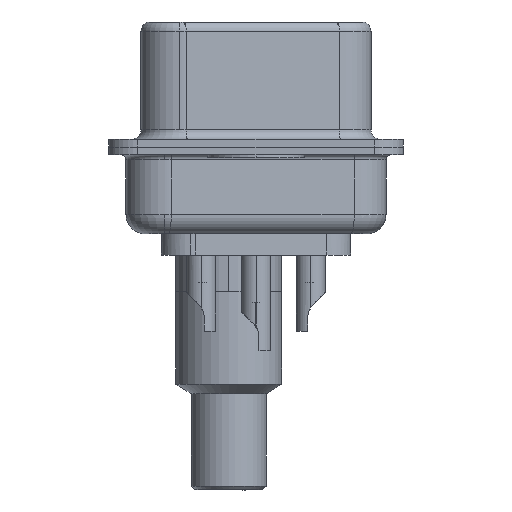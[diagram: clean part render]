
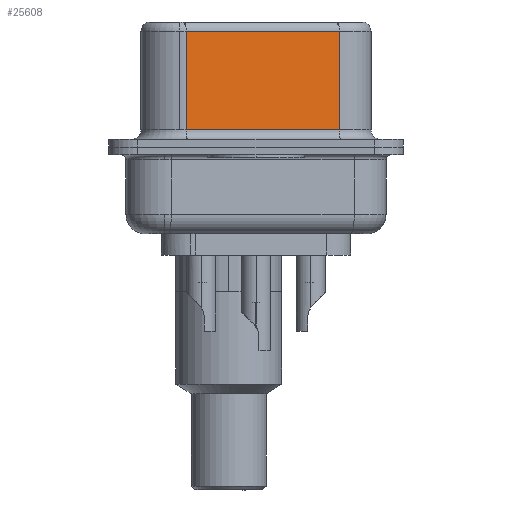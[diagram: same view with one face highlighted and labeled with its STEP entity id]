
A CAD part, left-side view. The second image highlights one B-rep face of the part: STEP entity #25608.
In plain terms, the highlighted planar face has unit normal (-0.985, -0.174, 0).
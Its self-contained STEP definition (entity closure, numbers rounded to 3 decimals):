
#132 = DIRECTION ( 'NONE',  ( 0., 0., -1. ) ) ;
#727 = EDGE_CURVE ( 'NONE', #9712, #7516, #27015, .T. ) ;
#1267 = VERTEX_POINT ( 'NONE', #26744 ) ;
#1799 = ORIENTED_EDGE ( 'NONE', *, *, #2211, .F. ) ;
#2211 = EDGE_CURVE ( 'NONE', #9136, #1267, #12298, .T. ) ;
#2888 = EDGE_CURVE ( 'NONE', #9136, #9712, #11550, .T. ) ;
#3516 = ORIENTED_EDGE ( 'NONE', *, *, #9710, .T. ) ;
#4111 = DIRECTION ( 'NONE',  ( 0.985, 0.174, 0. ) ) ;
#5671 = CARTESIAN_POINT ( 'NONE',  ( 5.132, -4.322, 0.9 ) ) ;
#6858 = LINE ( 'NONE', #5671, #7214 ) ;
#7164 = VECTOR ( 'NONE', #17624, 1000. ) ;
#7214 = VECTOR ( 'NONE', #22082, 1000. ) ;
#7516 = VERTEX_POINT ( 'NONE', #7781 ) ;
#7781 = CARTESIAN_POINT ( 'NONE',  ( 3.73, 3.628, 0.9 ) ) ;
#8131 = PLANE ( 'NONE',  #19898 ) ;
#8931 = DIRECTION ( 'NONE',  ( -0.174, 0.985, 0. ) ) ;
#9136 = VERTEX_POINT ( 'NONE', #16695 ) ;
#9710 = EDGE_CURVE ( 'NONE', #7516, #1267, #6858, .T. ) ;
#9712 = VERTEX_POINT ( 'NONE', #24383 ) ;
#9952 = CARTESIAN_POINT ( 'NONE',  ( 5.132, -4.322, 6.52 ) ) ;
#11550 = LINE ( 'NONE', #28993, #19394 ) ;
#12099 = DIRECTION ( 'NONE',  ( -0.174, 0.985, 0. ) ) ;
#12298 = LINE ( 'NONE', #9952, #27668 ) ;
#12645 = FACE_OUTER_BOUND ( 'NONE', #20928, .T. ) ;
#15538 = CARTESIAN_POINT ( 'NONE',  ( 3.73, 3.628, 6.52 ) ) ;
#16695 = CARTESIAN_POINT ( 'NONE',  ( 5.132, -4.322, 6.02 ) ) ;
#17624 = DIRECTION ( 'NONE',  ( 0., 0., -1. ) ) ;
#19394 = VECTOR ( 'NONE', #12099, 1000. ) ;
#19898 = AXIS2_PLACEMENT_3D ( 'NONE', #30472, #4111, #8931 ) ;
#20928 = EDGE_LOOP ( 'NONE', ( #1799, #23821, #30850, #3516 ) ) ;
#22082 = DIRECTION ( 'NONE',  ( 0.174, -0.985, 0. ) ) ;
#23821 = ORIENTED_EDGE ( 'NONE', *, *, #2888, .T. ) ;
#24383 = CARTESIAN_POINT ( 'NONE',  ( 3.73, 3.628, 6.02 ) ) ;
#25608 = ADVANCED_FACE ( 'NONE', ( #12645 ), #8131, .F. ) ;
#26744 = CARTESIAN_POINT ( 'NONE',  ( 5.132, -4.322, 0.9 ) ) ;
#27015 = LINE ( 'NONE', #15538, #7164 ) ;
#27668 = VECTOR ( 'NONE', #132, 1000. ) ;
#28993 = CARTESIAN_POINT ( 'NONE',  ( 5.132, -4.322, 6.02 ) ) ;
#30472 = CARTESIAN_POINT ( 'NONE',  ( 5.132, -4.322, 6.52 ) ) ;
#30850 = ORIENTED_EDGE ( 'NONE', *, *, #727, .T. ) ;
